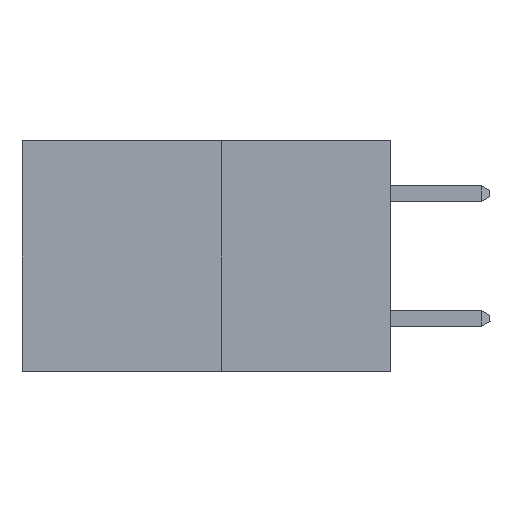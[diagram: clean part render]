
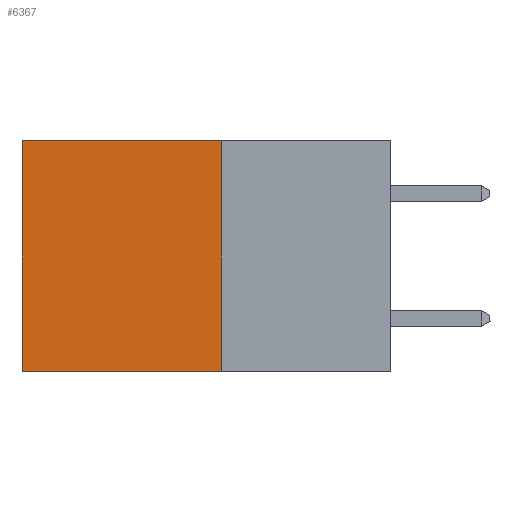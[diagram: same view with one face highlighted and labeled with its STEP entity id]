
A CAD part, left-side view. The second image highlights one B-rep face of the part: STEP entity #6367.
In plain terms, the highlighted planar face has unit normal (-1, 0, 0).
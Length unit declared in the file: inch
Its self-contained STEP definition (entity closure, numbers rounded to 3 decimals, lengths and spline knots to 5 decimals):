
#1414 = CARTESIAN_POINT ( 'NONE',  ( 0.277, 0.27, 0. ) ) ;
#1562 = LINE ( 'NONE', #8104, #17637 ) ;
#2132 = EDGE_CURVE ( 'NONE', #7776, #27459, #26420, .T. ) ;
#5744 = PLANE ( 'NONE',  #23801 ) ;
#6367 = ADVANCED_FACE ( 'NONE', ( #21615 ), #5744, .F. ) ;
#6691 = EDGE_CURVE ( 'NONE', #12007, #27459, #12396, .T. ) ;
#7266 = CARTESIAN_POINT ( 'NONE',  ( 0.277, 0.27, -0.37 ) ) ;
#7776 = VERTEX_POINT ( 'NONE', #23261 ) ;
#8104 = CARTESIAN_POINT ( 'NONE',  ( 0.277, 0.27, 0. ) ) ;
#8831 = CARTESIAN_POINT ( 'NONE',  ( 0.277, 0.27, -0.37 ) ) ;
#8967 = EDGE_LOOP ( 'NONE', ( #23325, #9913, #17150, #22617 ) ) ;
#9124 = EDGE_CURVE ( 'NONE', #13048, #7776, #22240, .T. ) ;
#9509 = DIRECTION ( 'NONE',  ( 0., 0., -1. ) ) ;
#9913 = ORIENTED_EDGE ( 'NONE', *, *, #2132, .F. ) ;
#10421 = DIRECTION ( 'NONE',  ( 0., 1., 0. ) ) ;
#12007 = VERTEX_POINT ( 'NONE', #15756 ) ;
#12396 = LINE ( 'NONE', #20298, #18377 ) ;
#13048 = VERTEX_POINT ( 'NONE', #1414 ) ;
#13670 = VECTOR ( 'NONE', #26563, 39.37008 ) ;
#14674 = CARTESIAN_POINT ( 'NONE',  ( 0.277, 0.59, -0.37 ) ) ;
#15756 = CARTESIAN_POINT ( 'NONE',  ( 0.277, 0.59, 0. ) ) ;
#15801 = DIRECTION ( 'NONE',  ( 1., 0., 0. ) ) ;
#17150 = ORIENTED_EDGE ( 'NONE', *, *, #9124, .F. ) ;
#17637 = VECTOR ( 'NONE', #10421, 39.37008 ) ;
#18099 = DIRECTION ( 'NONE',  ( 0., 0., -1. ) ) ;
#18377 = VECTOR ( 'NONE', #19743, 39.37008 ) ;
#18777 = EDGE_CURVE ( 'NONE', #13048, #12007, #1562, .T. ) ;
#19743 = DIRECTION ( 'NONE',  ( 0., 0., -1. ) ) ;
#20298 = CARTESIAN_POINT ( 'NONE',  ( 0.277, 0.59, -0.37 ) ) ;
#21615 = FACE_OUTER_BOUND ( 'NONE', #8967, .T. ) ;
#22240 = LINE ( 'NONE', #7266, #27521 ) ;
#22617 = ORIENTED_EDGE ( 'NONE', *, *, #18777, .T. ) ;
#22872 = CARTESIAN_POINT ( 'NONE',  ( 0.277, 0.27, -0.37 ) ) ;
#23261 = CARTESIAN_POINT ( 'NONE',  ( 0.277, 0.27, -0.37 ) ) ;
#23325 = ORIENTED_EDGE ( 'NONE', *, *, #6691, .T. ) ;
#23801 = AXIS2_PLACEMENT_3D ( 'NONE', #8831, #15801, #18099 ) ;
#26420 = LINE ( 'NONE', #22872, #13670 ) ;
#26563 = DIRECTION ( 'NONE',  ( 0., 1., 0. ) ) ;
#27459 = VERTEX_POINT ( 'NONE', #14674 ) ;
#27521 = VECTOR ( 'NONE', #9509, 39.37008 ) ;
